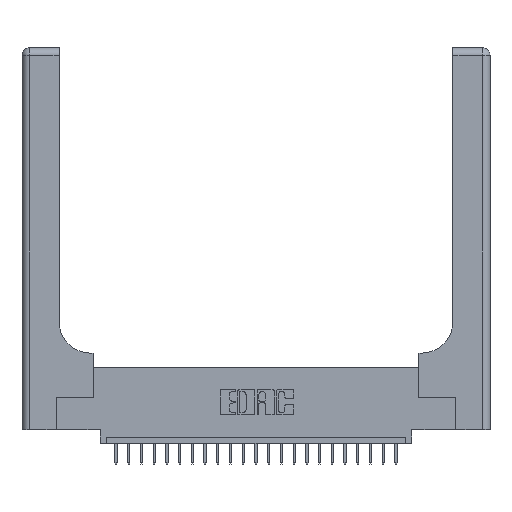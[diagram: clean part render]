
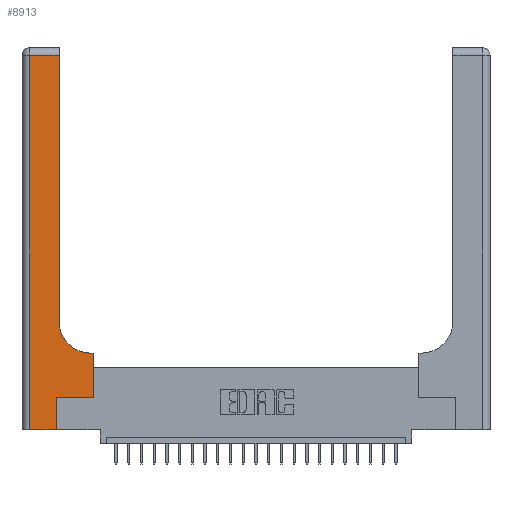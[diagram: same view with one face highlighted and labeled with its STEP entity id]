
A CAD part, top view. The second image highlights one B-rep face of the part: STEP entity #8913.
In plain terms, the highlighted planar face has unit normal (0, 0, 1).
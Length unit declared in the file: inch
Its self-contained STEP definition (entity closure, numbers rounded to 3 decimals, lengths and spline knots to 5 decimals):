
#127 = VECTOR ( 'NONE', #12381, 39.37008 ) ;
#186 = ORIENTED_EDGE ( 'NONE', *, *, #4885, .T. ) ;
#249 = DIRECTION ( 'NONE',  ( 0., 1., 0. ) ) ;
#952 = ORIENTED_EDGE ( 'NONE', *, *, #8570, .T. ) ;
#1228 = DIRECTION ( 'NONE',  ( 0., -1., 0. ) ) ;
#1662 = CARTESIAN_POINT ( 'NONE',  ( 0.5585, 0.25, 0.37 ) ) ;
#2431 = AXIS2_PLACEMENT_3D ( 'NONE', #12519, #9086, #24328 ) ;
#2514 = EDGE_CURVE ( 'NONE', #14278, #4319, #2801, .T. ) ;
#2583 = VECTOR ( 'NONE', #4718, 39.37008 ) ;
#2801 = LINE ( 'NONE', #12349, #17727 ) ;
#2872 = VECTOR ( 'NONE', #1228, 39.37008 ) ;
#3121 = EDGE_LOOP ( 'NONE', ( #13762, #22482, #952, #186, #12560, #20454, #6809, #4148, #11561 ) ) ;
#3184 = VERTEX_POINT ( 'NONE', #10924 ) ;
#3463 = EDGE_CURVE ( 'NONE', #13029, #12006, #19182, .T. ) ;
#4148 = ORIENTED_EDGE ( 'NONE', *, *, #4535, .T. ) ;
#4319 = VERTEX_POINT ( 'NONE', #19086 ) ;
#4535 = EDGE_CURVE ( 'NONE', #12006, #21908, #21254, .T. ) ;
#4712 = CARTESIAN_POINT ( 'NONE',  ( 0.2915, 0.6, 0.37 ) ) ;
#4718 = DIRECTION ( 'NONE',  ( 1., 0., 0. ) ) ;
#4809 = LINE ( 'NONE', #23183, #24879 ) ;
#4885 = EDGE_CURVE ( 'NONE', #24764, #21156, #24644, .T. ) ;
#4886 = CARTESIAN_POINT ( 'NONE',  ( 0.269, 0.25, 0.37 ) ) ;
#4993 = FACE_OUTER_BOUND ( 'NONE', #3121, .T. ) ;
#5024 = CARTESIAN_POINT ( 'NONE',  ( 0.06, 3., 0.37 ) ) ;
#5250 = CARTESIAN_POINT ( 'NONE',  ( 0.2915, 0.85, 0.37 ) ) ;
#5984 = EDGE_CURVE ( 'NONE', #13296, #14278, #4809, .T. ) ;
#6342 = CARTESIAN_POINT ( 'NONE',  ( 0.5585, 0.6, 0.37 ) ) ;
#6559 = CARTESIAN_POINT ( 'NONE',  ( 0., 0., 0.37 ) ) ;
#6809 = ORIENTED_EDGE ( 'NONE', *, *, #3463, .T. ) ;
#7102 = CARTESIAN_POINT ( 'NONE',  ( 0.5415, 0.85, 0.37 ) ) ;
#7162 = LINE ( 'NONE', #4886, #2583 ) ;
#7343 = EDGE_CURVE ( 'NONE', #21156, #3184, #23615, .T. ) ;
#7414 = CARTESIAN_POINT ( 'NONE',  ( 0.5415, 0.6, 0.37 ) ) ;
#8570 = EDGE_CURVE ( 'NONE', #4319, #24764, #18401, .T. ) ;
#8913 = ADVANCED_FACE ( 'NONE', ( #4993 ), #22266, .F. ) ;
#9086 = DIRECTION ( 'NONE',  ( 0., 0., -1. ) ) ;
#9106 = DIRECTION ( 'NONE',  ( 1., 0., 0. ) ) ;
#9545 = DIRECTION ( 'NONE',  ( 1., 0., 0. ) ) ;
#10924 = CARTESIAN_POINT ( 'NONE',  ( 0.269, 0.25, 0.37 ) ) ;
#11561 = ORIENTED_EDGE ( 'NONE', *, *, #11996, .T. ) ;
#11996 = EDGE_CURVE ( 'NONE', #21908, #13296, #19790, .T. ) ;
#12006 = VERTEX_POINT ( 'NONE', #6342 ) ;
#12131 = VECTOR ( 'NONE', #20363, 39.37008 ) ;
#12349 = CARTESIAN_POINT ( 'NONE',  ( 0., 2.94, 0.37 ) ) ;
#12381 = DIRECTION ( 'NONE',  ( 0., 1., 0. ) ) ;
#12519 = CARTESIAN_POINT ( 'NONE',  ( 0., 3., 0.37 ) ) ;
#12560 = ORIENTED_EDGE ( 'NONE', *, *, #7343, .T. ) ;
#12804 = VECTOR ( 'NONE', #17737, 39.37008 ) ;
#13029 = VERTEX_POINT ( 'NONE', #14163 ) ;
#13296 = VERTEX_POINT ( 'NONE', #5250 ) ;
#13762 = ORIENTED_EDGE ( 'NONE', *, *, #5984, .T. ) ;
#13925 = CARTESIAN_POINT ( 'NONE',  ( 0.06, 0., 0.37 ) ) ;
#14163 = CARTESIAN_POINT ( 'NONE',  ( 0.5585, 0.25, 0.37 ) ) ;
#14278 = VERTEX_POINT ( 'NONE', #24063 ) ;
#14878 = DIRECTION ( 'NONE',  ( -1., 0., 0. ) ) ;
#15721 = AXIS2_PLACEMENT_3D ( 'NONE', #7102, #24717, #9545 ) ;
#16740 = VECTOR ( 'NONE', #9106, 39.37008 ) ;
#17727 = VECTOR ( 'NONE', #14878, 39.37008 ) ;
#17737 = DIRECTION ( 'NONE',  ( 0., 1., 0. ) ) ;
#18401 = LINE ( 'NONE', #5024, #2872 ) ;
#18433 = CARTESIAN_POINT ( 'NONE',  ( 0.269, 0., 0.37 ) ) ;
#19086 = CARTESIAN_POINT ( 'NONE',  ( 0.06, 2.94, 0.37 ) ) ;
#19182 = LINE ( 'NONE', #1662, #12804 ) ;
#19790 = CIRCLE ( 'NONE', #15721, 0.25 ) ;
#20363 = DIRECTION ( 'NONE',  ( -1., 0., 0. ) ) ;
#20454 = ORIENTED_EDGE ( 'NONE', *, *, #21715, .T. ) ;
#21156 = VERTEX_POINT ( 'NONE', #18433 ) ;
#21254 = LINE ( 'NONE', #4712, #12131 ) ;
#21715 = EDGE_CURVE ( 'NONE', #3184, #13029, #7162, .T. ) ;
#21908 = VERTEX_POINT ( 'NONE', #7414 ) ;
#22266 = PLANE ( 'NONE',  #2431 ) ;
#22482 = ORIENTED_EDGE ( 'NONE', *, *, #2514, .T. ) ;
#23183 = CARTESIAN_POINT ( 'NONE',  ( 0.2915, 3., 0.37 ) ) ;
#23615 = LINE ( 'NONE', #24011, #127 ) ;
#24011 = CARTESIAN_POINT ( 'NONE',  ( 0.269, 0., 0.37 ) ) ;
#24063 = CARTESIAN_POINT ( 'NONE',  ( 0.2915, 2.94, 0.37 ) ) ;
#24328 = DIRECTION ( 'NONE',  ( -1., 0., 0. ) ) ;
#24644 = LINE ( 'NONE', #6559, #16740 ) ;
#24717 = DIRECTION ( 'NONE',  ( 0., 0., -1. ) ) ;
#24764 = VERTEX_POINT ( 'NONE', #13925 ) ;
#24879 = VECTOR ( 'NONE', #249, 39.37008 ) ;
